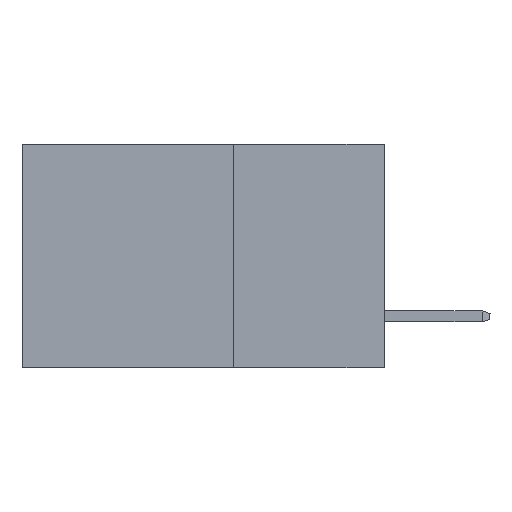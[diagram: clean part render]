
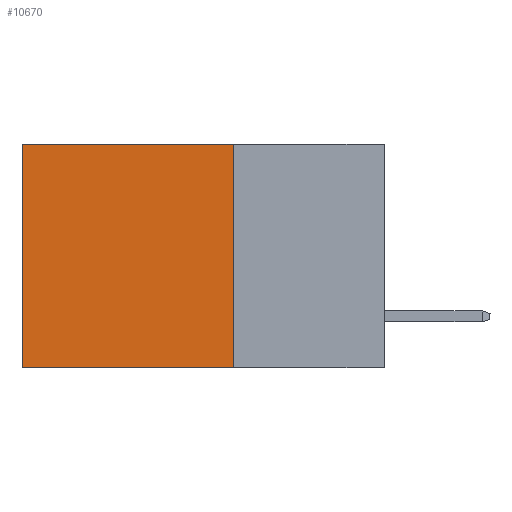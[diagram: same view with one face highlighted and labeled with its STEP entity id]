
A CAD part, left-side view. The second image highlights one B-rep face of the part: STEP entity #10670.
In plain terms, the highlighted planar face has unit normal (-1, 0, 0).
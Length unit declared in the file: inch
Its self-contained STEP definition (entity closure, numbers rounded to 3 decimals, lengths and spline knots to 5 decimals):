
#195 = DIRECTION ( 'NONE',  ( 0., 1., 0. ) ) ;
#560 = ORIENTED_EDGE ( 'NONE', *, *, #22738, .F. ) ;
#1287 = VERTEX_POINT ( 'NONE', #7642 ) ;
#2760 = DIRECTION ( 'NONE',  ( 1., 0., 0. ) ) ;
#4015 = VECTOR ( 'NONE', #24060, 39.37008 ) ;
#4291 = ORIENTED_EDGE ( 'NONE', *, *, #12178, .T. ) ;
#4357 = LINE ( 'NONE', #18930, #11206 ) ;
#4484 = FACE_OUTER_BOUND ( 'NONE', #13460, .T. ) ;
#4842 = DIRECTION ( 'NONE',  ( 0., 0., -1. ) ) ;
#5204 = CARTESIAN_POINT ( 'NONE',  ( 0.2615, 0.6, -0.37 ) ) ;
#5816 = EDGE_CURVE ( 'NONE', #10405, #15435, #18432, .T. ) ;
#6170 = ORIENTED_EDGE ( 'NONE', *, *, #5816, .T. ) ;
#6432 = AXIS2_PLACEMENT_3D ( 'NONE', #23089, #2760, #4842 ) ;
#6705 = LINE ( 'NONE', #10590, #15488 ) ;
#6940 = DIRECTION ( 'NONE',  ( 0., 1., 0. ) ) ;
#7265 = CARTESIAN_POINT ( 'NONE',  ( 0.2615, 0.25, 0. ) ) ;
#7642 = CARTESIAN_POINT ( 'NONE',  ( 0.2615, 0.25, 0. ) ) ;
#9490 = VERTEX_POINT ( 'NONE', #18860 ) ;
#10405 = VERTEX_POINT ( 'NONE', #10946 ) ;
#10575 = ORIENTED_EDGE ( 'NONE', *, *, #17111, .F. ) ;
#10590 = CARTESIAN_POINT ( 'NONE',  ( 0.2615, 0.25, -0.37 ) ) ;
#10670 = ADVANCED_FACE ( 'NONE', ( #4484 ), #11881, .F. ) ;
#10946 = CARTESIAN_POINT ( 'NONE',  ( 0.2615, 0.6, 0. ) ) ;
#11206 = VECTOR ( 'NONE', #19169, 39.37008 ) ;
#11881 = PLANE ( 'NONE',  #6432 ) ;
#12178 = EDGE_CURVE ( 'NONE', #1287, #10405, #23950, .T. ) ;
#13460 = EDGE_LOOP ( 'NONE', ( #6170, #10575, #560, #4291 ) ) ;
#15435 = VERTEX_POINT ( 'NONE', #18010 ) ;
#15488 = VECTOR ( 'NONE', #6940, 39.37008 ) ;
#16565 = VECTOR ( 'NONE', #195, 39.37008 ) ;
#17111 = EDGE_CURVE ( 'NONE', #9490, #15435, #6705, .T. ) ;
#18010 = CARTESIAN_POINT ( 'NONE',  ( 0.2615, 0.6, -0.37 ) ) ;
#18432 = LINE ( 'NONE', #5204, #4015 ) ;
#18860 = CARTESIAN_POINT ( 'NONE',  ( 0.2615, 0.25, -0.37 ) ) ;
#18930 = CARTESIAN_POINT ( 'NONE',  ( 0.2615, 0.25, -0.37 ) ) ;
#19169 = DIRECTION ( 'NONE',  ( 0., 0., -1. ) ) ;
#22738 = EDGE_CURVE ( 'NONE', #1287, #9490, #4357, .T. ) ;
#23089 = CARTESIAN_POINT ( 'NONE',  ( 0.2615, 0.25, -0.37 ) ) ;
#23950 = LINE ( 'NONE', #7265, #16565 ) ;
#24060 = DIRECTION ( 'NONE',  ( 0., 0., -1. ) ) ;
